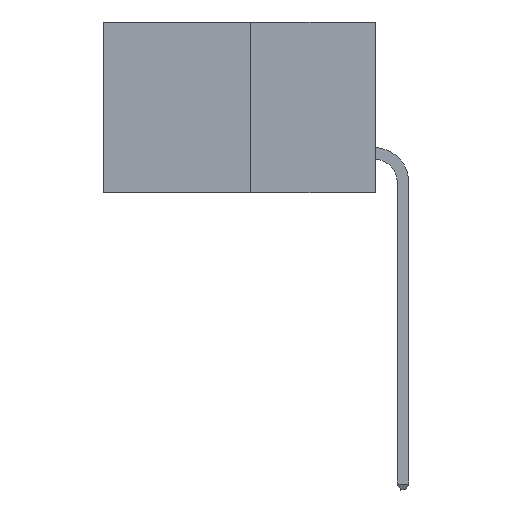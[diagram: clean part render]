
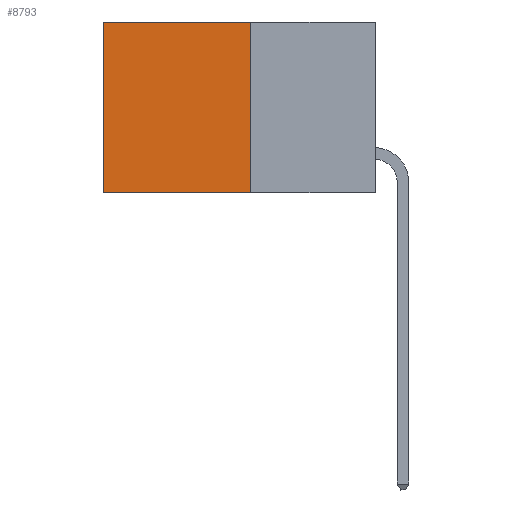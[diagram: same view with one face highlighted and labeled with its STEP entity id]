
A CAD part, left-side view. The second image highlights one B-rep face of the part: STEP entity #8793.
In plain terms, the highlighted planar face has unit normal (-1, 0, 0).
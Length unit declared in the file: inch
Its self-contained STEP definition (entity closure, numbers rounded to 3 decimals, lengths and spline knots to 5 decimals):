
#196 = CARTESIAN_POINT ( 'NONE',  ( 0.277, 0.27, 0. ) ) ;
#624 = EDGE_CURVE ( 'NONE', #3720, #12907, #9121, .T. ) ;
#1678 = CARTESIAN_POINT ( 'NONE',  ( 0.277, 0.27, 0. ) ) ;
#1684 = ORIENTED_EDGE ( 'NONE', *, *, #10263, .F. ) ;
#2041 = DIRECTION ( 'NONE',  ( 0., 1., 0. ) ) ;
#2181 = ORIENTED_EDGE ( 'NONE', *, *, #3856, .T. ) ;
#2736 = VERTEX_POINT ( 'NONE', #196 ) ;
#2757 = AXIS2_PLACEMENT_3D ( 'NONE', #5165, #12246, #6207 ) ;
#3097 = EDGE_CURVE ( 'NONE', #2736, #8051, #9072, .T. ) ;
#3720 = VERTEX_POINT ( 'NONE', #4371 ) ;
#3856 = EDGE_CURVE ( 'NONE', #8051, #12907, #11121, .T. ) ;
#4342 = FACE_OUTER_BOUND ( 'NONE', #10631, .T. ) ;
#4371 = CARTESIAN_POINT ( 'NONE',  ( 0.277, 0.27, -0.37 ) ) ;
#4889 = DIRECTION ( 'NONE',  ( 0., 1., 0. ) ) ;
#5165 = CARTESIAN_POINT ( 'NONE',  ( 0.277, 0.27, -0.37 ) ) ;
#5507 = CARTESIAN_POINT ( 'NONE',  ( 0.277, 0.27, -0.37 ) ) ;
#5644 = CARTESIAN_POINT ( 'NONE',  ( 0.277, 0.59, -0.37 ) ) ;
#5942 = ORIENTED_EDGE ( 'NONE', *, *, #624, .F. ) ;
#6207 = DIRECTION ( 'NONE',  ( 0., 0., -1. ) ) ;
#7678 = VECTOR ( 'NONE', #8517, 39.37008 ) ;
#8051 = VERTEX_POINT ( 'NONE', #8095 ) ;
#8095 = CARTESIAN_POINT ( 'NONE',  ( 0.277, 0.59, 0. ) ) ;
#8392 = VECTOR ( 'NONE', #9711, 39.37008 ) ;
#8517 = DIRECTION ( 'NONE',  ( 0., 0., -1. ) ) ;
#8748 = VECTOR ( 'NONE', #2041, 39.37008 ) ;
#8793 = ADVANCED_FACE ( 'NONE', ( #4342 ), #11259, .F. ) ;
#8794 = VECTOR ( 'NONE', #4889, 39.37008 ) ;
#9072 = LINE ( 'NONE', #1678, #8748 ) ;
#9121 = LINE ( 'NONE', #13108, #8794 ) ;
#9711 = DIRECTION ( 'NONE',  ( 0., 0., -1. ) ) ;
#10068 = LINE ( 'NONE', #5507, #7678 ) ;
#10263 = EDGE_CURVE ( 'NONE', #2736, #3720, #10068, .T. ) ;
#10520 = ORIENTED_EDGE ( 'NONE', *, *, #3097, .T. ) ;
#10631 = EDGE_LOOP ( 'NONE', ( #2181, #5942, #1684, #10520 ) ) ;
#11121 = LINE ( 'NONE', #5644, #8392 ) ;
#11259 = PLANE ( 'NONE',  #2757 ) ;
#11580 = CARTESIAN_POINT ( 'NONE',  ( 0.277, 0.59, -0.37 ) ) ;
#12246 = DIRECTION ( 'NONE',  ( 1., 0., 0. ) ) ;
#12907 = VERTEX_POINT ( 'NONE', #11580 ) ;
#13108 = CARTESIAN_POINT ( 'NONE',  ( 0.277, 0.27, -0.37 ) ) ;
